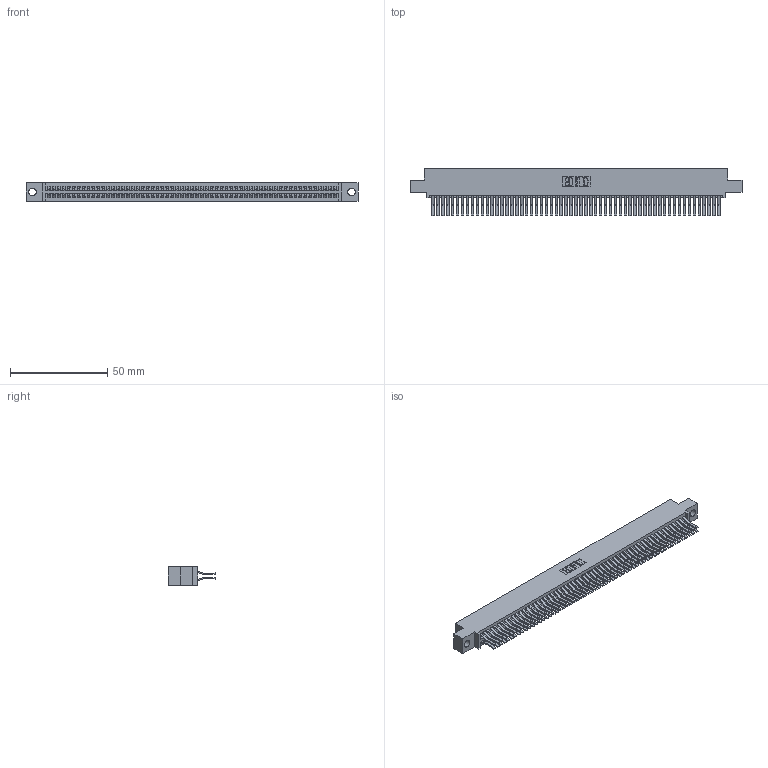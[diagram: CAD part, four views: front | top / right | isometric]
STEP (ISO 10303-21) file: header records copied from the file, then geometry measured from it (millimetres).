
FILE_DESCRIPTION (( 'STEP AP203' ), '1' );
FILE_NAME ('845-118-560-504.STEP', '2018-11-21T00:09:57', ( '' ), ( '' ), 'SwSTEP 2.0', 'SolidWorks 2016', '' );
FILE_SCHEMA (( 'CONFIG_CONTROL_DESIGN' ));
Length unit declared in the file: inch
Products named in the file (3): 845 Part_0.110 Offset - 0.156 Dia-TH; 345-292-001_560 Tail; 845-118-560-504
Assembly tree (119 placements, depth 2):
  845-118-560-504
    845 Part_0.110 Offset - 0.156 Dia-TH
    345-292-001_560 Tail  x118
Bounding box: 171.07 x 24.45 x 9.4 mm (x, y, z)
Volume: 17387.8 mm3; surface area: 27928.6 mm2
Topology: 119 solids, 119 shells, 6266 faces, 18643 edges, 12270 vertices
Faces by surface type: plane 3978, cylinder 2288
Entity records: 44227 total; most frequent: CARTESIAN_POINT 7400, ORIENTED_EDGE 7334, DIRECTION 6507, EDGE_CURVE 3667, LINE 3295, VECTOR 3295, VERTEX_POINT 2442, AXIS2_PLACEMENT_3D 1606
